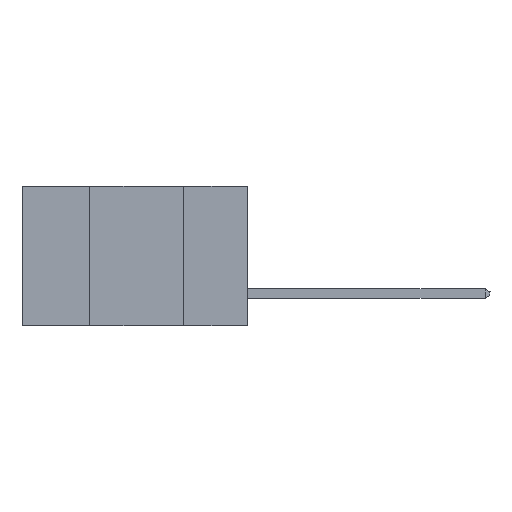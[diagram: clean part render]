
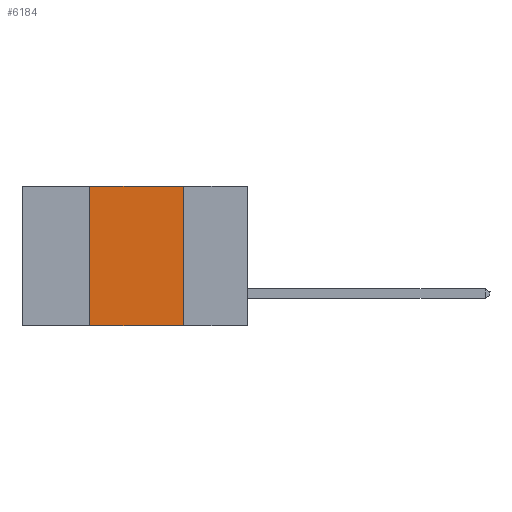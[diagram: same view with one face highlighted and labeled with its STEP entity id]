
A CAD part, left-side view. The second image highlights one B-rep face of the part: STEP entity #6184.
In plain terms, the highlighted planar face has unit normal (-1, 0, 0).
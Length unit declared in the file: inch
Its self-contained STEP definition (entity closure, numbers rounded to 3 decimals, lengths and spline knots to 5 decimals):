
#419 = DIRECTION ( 'NONE',  ( 0., 0., -1. ) ) ;
#757 = VECTOR ( 'NONE', #7896, 39.37008 ) ;
#1242 = CARTESIAN_POINT ( 'NONE',  ( 0., 0.6, -0.37 ) ) ;
#1513 = VERTEX_POINT ( 'NONE', #5736 ) ;
#1915 = LINE ( 'NONE', #4732, #9735 ) ;
#2218 = EDGE_LOOP ( 'NONE', ( #2312, #9734, #9766, #8690 ) ) ;
#2312 = ORIENTED_EDGE ( 'NONE', *, *, #4084, .F. ) ;
#2339 = CARTESIAN_POINT ( 'NONE',  ( 0., 0.17, -0.37 ) ) ;
#2421 = FACE_OUTER_BOUND ( 'NONE', #2218, .T. ) ;
#3019 = EDGE_CURVE ( 'NONE', #9909, #1513, #8280, .T. ) ;
#3244 = VERTEX_POINT ( 'NONE', #10731 ) ;
#4084 = EDGE_CURVE ( 'NONE', #1513, #3244, #4405, .T. ) ;
#4360 = CARTESIAN_POINT ( 'NONE',  ( 0., 0.42, -0.37 ) ) ;
#4405 = LINE ( 'NONE', #2339, #6066 ) ;
#4732 = CARTESIAN_POINT ( 'NONE',  ( 0., 0.42, -0.37 ) ) ;
#5047 = EDGE_CURVE ( 'NONE', #10727, #3244, #6014, .T. ) ;
#5274 = CARTESIAN_POINT ( 'NONE',  ( 0., 0.6, 0. ) ) ;
#5736 = CARTESIAN_POINT ( 'NONE',  ( 0., 0.17, 0. ) ) ;
#6014 = LINE ( 'NONE', #1242, #757 ) ;
#6066 = VECTOR ( 'NONE', #419, 39.37008 ) ;
#6184 = ADVANCED_FACE ( 'NONE', ( #2421 ), #8058, .F. ) ;
#7311 = DIRECTION ( 'NONE',  ( 0., -1., 0. ) ) ;
#7896 = DIRECTION ( 'NONE',  ( 0., -1., 0. ) ) ;
#7907 = AXIS2_PLACEMENT_3D ( 'NONE', #5274, #10587, #8004 ) ;
#8004 = DIRECTION ( 'NONE',  ( 0., 0., -1. ) ) ;
#8058 = PLANE ( 'NONE',  #7907 ) ;
#8280 = LINE ( 'NONE', #10133, #8355 ) ;
#8355 = VECTOR ( 'NONE', #7311, 39.37008 ) ;
#8483 = DIRECTION ( 'NONE',  ( 0., 0., 1. ) ) ;
#8690 = ORIENTED_EDGE ( 'NONE', *, *, #5047, .T. ) ;
#9734 = ORIENTED_EDGE ( 'NONE', *, *, #3019, .F. ) ;
#9735 = VECTOR ( 'NONE', #8483, 39.37008 ) ;
#9766 = ORIENTED_EDGE ( 'NONE', *, *, #10519, .F. ) ;
#9909 = VERTEX_POINT ( 'NONE', #11324 ) ;
#10133 = CARTESIAN_POINT ( 'NONE',  ( 0., 0.6, 0. ) ) ;
#10519 = EDGE_CURVE ( 'NONE', #10727, #9909, #1915, .T. ) ;
#10587 = DIRECTION ( 'NONE',  ( 1., 0., 0. ) ) ;
#10727 = VERTEX_POINT ( 'NONE', #4360 ) ;
#10731 = CARTESIAN_POINT ( 'NONE',  ( 0., 0.17, -0.37 ) ) ;
#11324 = CARTESIAN_POINT ( 'NONE',  ( 0., 0.42, 0. ) ) ;
